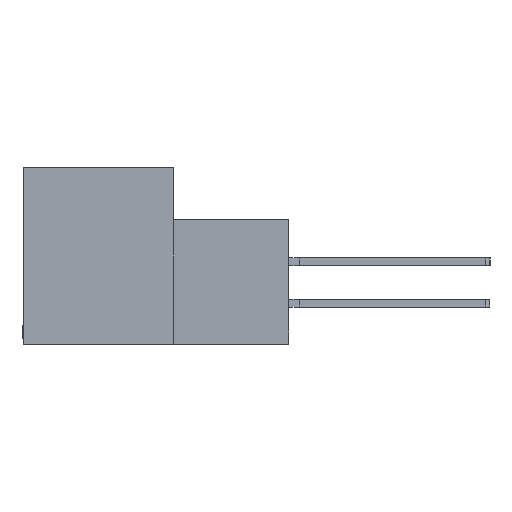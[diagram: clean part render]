
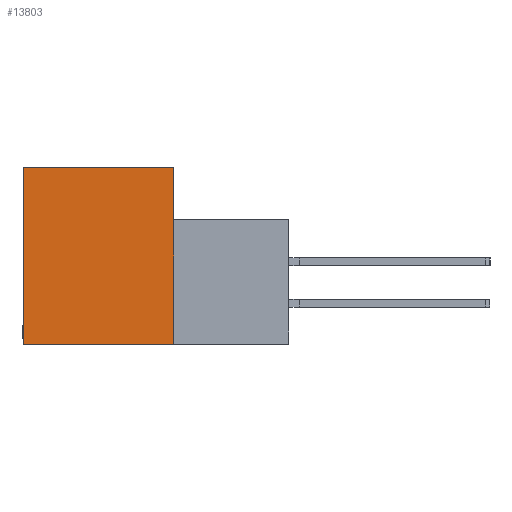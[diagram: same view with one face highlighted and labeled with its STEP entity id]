
A CAD part, left-side view. The second image highlights one B-rep face of the part: STEP entity #13803.
In plain terms, the highlighted planar face has unit normal (-1, 0, 0).
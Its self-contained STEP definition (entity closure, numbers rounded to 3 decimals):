
#409 = CARTESIAN_POINT ( 'NONE',  ( 0., -8.814, -13.487 ) ) ;
#1960 = VECTOR ( 'NONE', #5324, 1000. ) ;
#2997 = CARTESIAN_POINT ( 'NONE',  ( 0., 0., 0. ) ) ;
#3846 = CARTESIAN_POINT ( 'NONE',  ( 0., 11.506, -13.487 ) ) ;
#4015 = ORIENTED_EDGE ( 'NONE', *, *, #17780, .F. ) ;
#4424 = EDGE_CURVE ( 'NONE', #23469, #5721, #23485, .T. ) ;
#5260 = DIRECTION ( 'NONE',  ( 0., 0., -1. ) ) ;
#5324 = DIRECTION ( 'NONE',  ( 0., 0., -1. ) ) ;
#5721 = VERTEX_POINT ( 'NONE', #24138 ) ;
#6056 = EDGE_LOOP ( 'NONE', ( #15698, #22634, #4015, #24887 ) ) ;
#6495 = VECTOR ( 'NONE', #25029, 1000. ) ;
#9703 = PLANE ( 'NONE',  #27012 ) ;
#10777 = DIRECTION ( 'NONE',  ( 0., 0., 1. ) ) ;
#11266 = VERTEX_POINT ( 'NONE', #28279 ) ;
#11498 = EDGE_CURVE ( 'NONE', #20763, #11266, #17166, .T. ) ;
#11770 = FACE_OUTER_BOUND ( 'NONE', #6056, .T. ) ;
#12053 = CARTESIAN_POINT ( 'NONE',  ( 0., 0., 0. ) ) ;
#12358 = CARTESIAN_POINT ( 'NONE',  ( 0., 11.506, 0. ) ) ;
#13803 = ADVANCED_FACE ( 'NONE', ( #11770 ), #9703, .F. ) ;
#14641 = DIRECTION ( 'NONE',  ( 0., -1., 0. ) ) ;
#15698 = ORIENTED_EDGE ( 'NONE', *, *, #23954, .F. ) ;
#16108 = CARTESIAN_POINT ( 'NONE',  ( 0., 0., 0. ) ) ;
#17109 = LINE ( 'NONE', #409, #6495 ) ;
#17166 = LINE ( 'NONE', #12053, #1960 ) ;
#17780 = EDGE_CURVE ( 'NONE', #5721, #20763, #17943, .T. ) ;
#17943 = LINE ( 'NONE', #12358, #20055 ) ;
#18805 = DIRECTION ( 'NONE',  ( 1., 0., 0. ) ) ;
#20055 = VECTOR ( 'NONE', #14641, 1000. ) ;
#20489 = CARTESIAN_POINT ( 'NONE',  ( 0., 11.506, -13.487 ) ) ;
#20763 = VERTEX_POINT ( 'NONE', #16108 ) ;
#22634 = ORIENTED_EDGE ( 'NONE', *, *, #11498, .F. ) ;
#23469 = VERTEX_POINT ( 'NONE', #20489 ) ;
#23485 = LINE ( 'NONE', #3846, #27385 ) ;
#23954 = EDGE_CURVE ( 'NONE', #11266, #23469, #17109, .T. ) ;
#24138 = CARTESIAN_POINT ( 'NONE',  ( 0., 11.506, 0. ) ) ;
#24887 = ORIENTED_EDGE ( 'NONE', *, *, #4424, .F. ) ;
#25029 = DIRECTION ( 'NONE',  ( 0., 1., 0. ) ) ;
#27012 = AXIS2_PLACEMENT_3D ( 'NONE', #2997, #18805, #5260 ) ;
#27385 = VECTOR ( 'NONE', #10777, 1000. ) ;
#28279 = CARTESIAN_POINT ( 'NONE',  ( 0., 0., -13.487 ) ) ;
